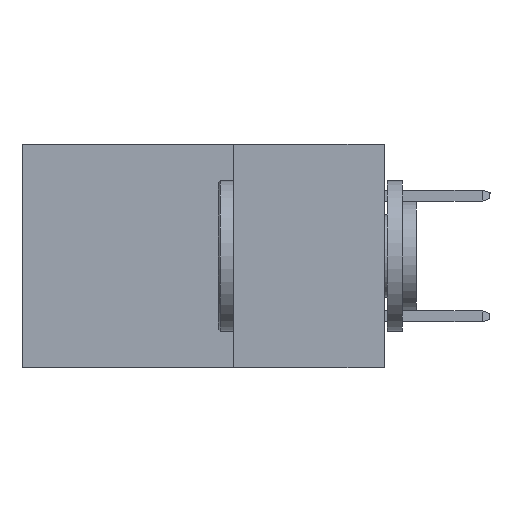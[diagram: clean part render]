
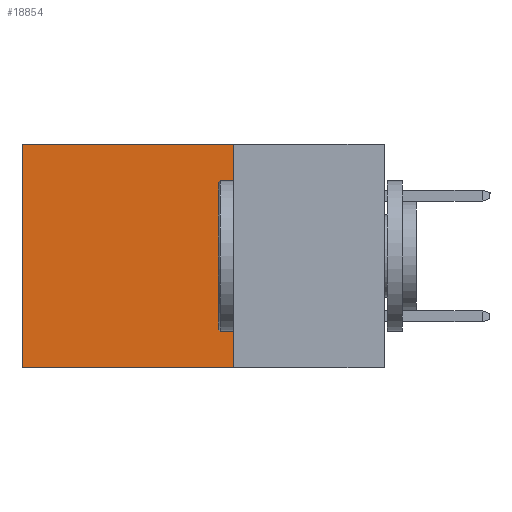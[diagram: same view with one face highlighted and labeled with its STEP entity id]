
A CAD part, left-side view. The second image highlights one B-rep face of the part: STEP entity #18854.
In plain terms, the highlighted planar face has unit normal (-1, 0, 0).
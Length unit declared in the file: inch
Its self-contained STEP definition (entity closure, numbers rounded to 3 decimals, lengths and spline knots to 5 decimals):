
#265 = ORIENTED_EDGE ( 'NONE', *, *, #10685, .F. ) ;
#331 = DIRECTION ( 'NONE',  ( 0., 0., -1. ) ) ;
#536 = ORIENTED_EDGE ( 'NONE', *, *, #11059, .T. ) ;
#731 = EDGE_CURVE ( 'NONE', #9065, #6903, #6799, .T. ) ;
#885 = DIRECTION ( 'NONE',  ( 0., 0., -1. ) ) ;
#1025 = DIRECTION ( 'NONE',  ( 0., 1., 0. ) ) ;
#1060 = CARTESIAN_POINT ( 'NONE',  ( 0.2615, 0.25, 0. ) ) ;
#1508 = ORIENTED_EDGE ( 'NONE', *, *, #731, .F. ) ;
#1793 = VERTEX_POINT ( 'NONE', #1060 ) ;
#2291 = LINE ( 'NONE', #22446, #24199 ) ;
#3020 = CARTESIAN_POINT ( 'NONE',  ( 0.2615, 0.25, -0.37 ) ) ;
#4695 = LINE ( 'NONE', #7391, #24586 ) ;
#6799 = LINE ( 'NONE', #3020, #12734 ) ;
#6903 = VERTEX_POINT ( 'NONE', #17943 ) ;
#7391 = CARTESIAN_POINT ( 'NONE',  ( 0.2615, 0.25, -0.37 ) ) ;
#7839 = VECTOR ( 'NONE', #10402, 39.37008 ) ;
#8336 = CARTESIAN_POINT ( 'NONE',  ( 0.2615, 0.25, 0. ) ) ;
#8805 = DIRECTION ( 'NONE',  ( 1., 0., 0. ) ) ;
#9065 = VERTEX_POINT ( 'NONE', #22000 ) ;
#10173 = CARTESIAN_POINT ( 'NONE',  ( 0.2615, 0.6, 0. ) ) ;
#10402 = DIRECTION ( 'NONE',  ( 0., 1., 0. ) ) ;
#10685 = EDGE_CURVE ( 'NONE', #1793, #9065, #4695, .T. ) ;
#11059 = EDGE_CURVE ( 'NONE', #11956, #6903, #2291, .T. ) ;
#11956 = VERTEX_POINT ( 'NONE', #10173 ) ;
#12438 = DIRECTION ( 'NONE',  ( 0., 0., -1. ) ) ;
#12506 = EDGE_LOOP ( 'NONE', ( #536, #1508, #265, #24100 ) ) ;
#12734 = VECTOR ( 'NONE', #1025, 39.37008 ) ;
#17943 = CARTESIAN_POINT ( 'NONE',  ( 0.2615, 0.6, -0.37 ) ) ;
#18151 = CARTESIAN_POINT ( 'NONE',  ( 0.2615, 0.25, -0.37 ) ) ;
#18854 = ADVANCED_FACE ( 'NONE', ( #24156 ), #24423, .F. ) ;
#18975 = EDGE_CURVE ( 'NONE', #1793, #11956, #24067, .T. ) ;
#22000 = CARTESIAN_POINT ( 'NONE',  ( 0.2615, 0.25, -0.37 ) ) ;
#22446 = CARTESIAN_POINT ( 'NONE',  ( 0.2615, 0.6, -0.37 ) ) ;
#23681 = AXIS2_PLACEMENT_3D ( 'NONE', #18151, #8805, #331 ) ;
#24067 = LINE ( 'NONE', #8336, #7839 ) ;
#24100 = ORIENTED_EDGE ( 'NONE', *, *, #18975, .T. ) ;
#24156 = FACE_OUTER_BOUND ( 'NONE', #12506, .T. ) ;
#24199 = VECTOR ( 'NONE', #12438, 39.37008 ) ;
#24423 = PLANE ( 'NONE',  #23681 ) ;
#24586 = VECTOR ( 'NONE', #885, 39.37008 ) ;
